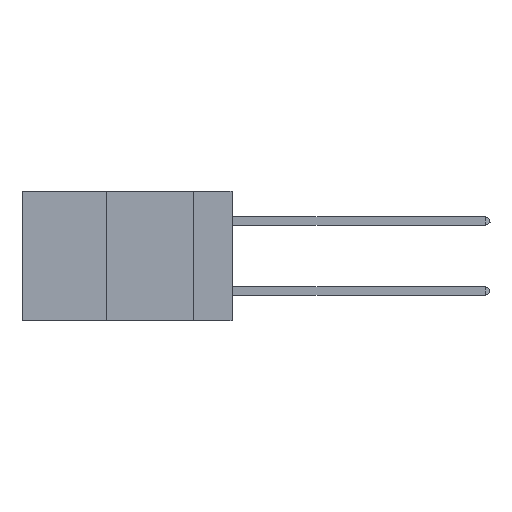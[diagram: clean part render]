
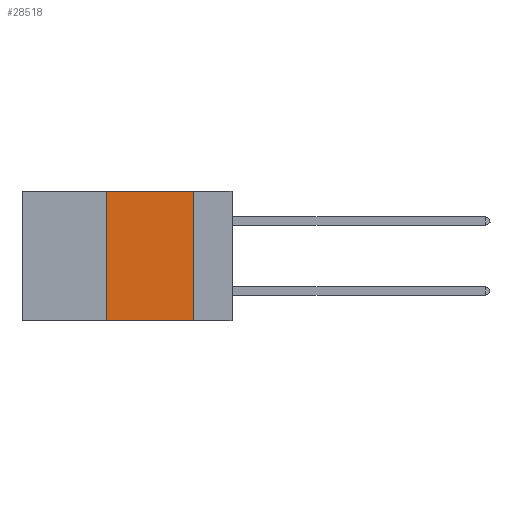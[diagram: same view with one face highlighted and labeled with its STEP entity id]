
A CAD part, left-side view. The second image highlights one B-rep face of the part: STEP entity #28518.
In plain terms, the highlighted planar face has unit normal (-1, 0, 0).
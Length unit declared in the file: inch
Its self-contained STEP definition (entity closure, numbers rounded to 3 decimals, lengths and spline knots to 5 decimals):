
#1247 = FACE_OUTER_BOUND ( 'NONE', #33456, .T. ) ;
#3212 = ORIENTED_EDGE ( 'NONE', *, *, #8242, .F. ) ;
#5334 = CARTESIAN_POINT ( 'NONE',  ( 0., 0.6, 0. ) ) ;
#5722 = CARTESIAN_POINT ( 'NONE',  ( 0., 0.36, -0.37 ) ) ;
#5916 = CARTESIAN_POINT ( 'NONE',  ( 0., 0.11, -0.37 ) ) ;
#6010 = LINE ( 'NONE', #19341, #10763 ) ;
#7161 = AXIS2_PLACEMENT_3D ( 'NONE', #32950, #11805, #24812 ) ;
#8242 = EDGE_CURVE ( 'NONE', #25625, #16738, #29055, .T. ) ;
#9182 = VERTEX_POINT ( 'NONE', #5722 ) ;
#9472 = CARTESIAN_POINT ( 'NONE',  ( 0., 0.11, 0. ) ) ;
#10763 = VECTOR ( 'NONE', #16064, 39.37008 ) ;
#11324 = VECTOR ( 'NONE', #20128, 39.37008 ) ;
#11805 = DIRECTION ( 'NONE',  ( 1., 0., 0. ) ) ;
#11881 = ORIENTED_EDGE ( 'NONE', *, *, #12825, .T. ) ;
#12825 = EDGE_CURVE ( 'NONE', #9182, #27180, #33633, .T. ) ;
#13638 = DIRECTION ( 'NONE',  ( 0., -1., 0. ) ) ;
#14422 = CARTESIAN_POINT ( 'NONE',  ( 0., 0.6, -0.37 ) ) ;
#14991 = ORIENTED_EDGE ( 'NONE', *, *, #21235, .F. ) ;
#16064 = DIRECTION ( 'NONE',  ( 0., 0., -1. ) ) ;
#16738 = VERTEX_POINT ( 'NONE', #9472 ) ;
#19341 = CARTESIAN_POINT ( 'NONE',  ( 0., 0.11, 0. ) ) ;
#19712 = CARTESIAN_POINT ( 'NONE',  ( 0., 0.36, 0. ) ) ;
#20128 = DIRECTION ( 'NONE',  ( 0., -1., 0. ) ) ;
#21235 = EDGE_CURVE ( 'NONE', #16738, #27180, #6010, .T. ) ;
#21415 = VECTOR ( 'NONE', #24742, 39.37008 ) ;
#24701 = EDGE_CURVE ( 'NONE', #9182, #25625, #30106, .T. ) ;
#24742 = DIRECTION ( 'NONE',  ( 0., 0., 1. ) ) ;
#24812 = DIRECTION ( 'NONE',  ( 0., 0., -1. ) ) ;
#25625 = VERTEX_POINT ( 'NONE', #30321 ) ;
#26862 = ORIENTED_EDGE ( 'NONE', *, *, #24701, .F. ) ;
#27180 = VERTEX_POINT ( 'NONE', #5916 ) ;
#27740 = PLANE ( 'NONE',  #7161 ) ;
#28518 = ADVANCED_FACE ( 'NONE', ( #1247 ), #27740, .F. ) ;
#29055 = LINE ( 'NONE', #5334, #33896 ) ;
#30106 = LINE ( 'NONE', #19712, #21415 ) ;
#30321 = CARTESIAN_POINT ( 'NONE',  ( 0., 0.36, 0. ) ) ;
#32950 = CARTESIAN_POINT ( 'NONE',  ( 0., 0.6, 0. ) ) ;
#33456 = EDGE_LOOP ( 'NONE', ( #14991, #3212, #26862, #11881 ) ) ;
#33633 = LINE ( 'NONE', #14422, #11324 ) ;
#33896 = VECTOR ( 'NONE', #13638, 39.37008 ) ;
